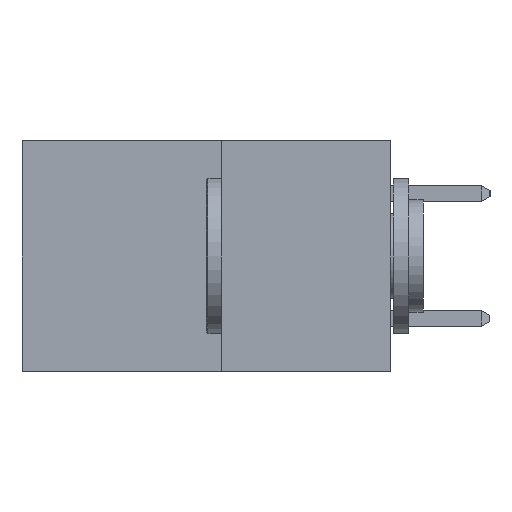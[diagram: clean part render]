
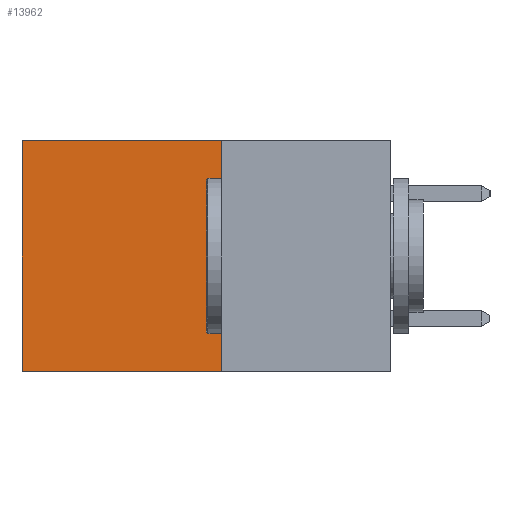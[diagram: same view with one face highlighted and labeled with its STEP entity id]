
A CAD part, left-side view. The second image highlights one B-rep face of the part: STEP entity #13962.
In plain terms, the highlighted planar face has unit normal (-1, 0, 0).
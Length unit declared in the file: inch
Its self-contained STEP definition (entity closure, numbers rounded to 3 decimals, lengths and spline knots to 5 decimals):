
#373 = PLANE ( 'NONE',  #20520 ) ;
#533 = LINE ( 'NONE', #15297, #5423 ) ;
#648 = DIRECTION ( 'NONE',  ( 0., 1., 0. ) ) ;
#1032 = CARTESIAN_POINT ( 'NONE',  ( 0.277, 0.27, -0.37 ) ) ;
#1440 = CARTESIAN_POINT ( 'NONE',  ( 0.277, 0.27, -0.37 ) ) ;
#1794 = ORIENTED_EDGE ( 'NONE', *, *, #9398, .F. ) ;
#2177 = VERTEX_POINT ( 'NONE', #14330 ) ;
#2356 = VECTOR ( 'NONE', #13836, 39.37008 ) ;
#4237 = VERTEX_POINT ( 'NONE', #17198 ) ;
#4848 = ORIENTED_EDGE ( 'NONE', *, *, #15363, .T. ) ;
#5423 = VECTOR ( 'NONE', #17040, 39.37008 ) ;
#5927 = DIRECTION ( 'NONE',  ( 1., 0., 0. ) ) ;
#6181 = EDGE_LOOP ( 'NONE', ( #23161, #22148, #1794, #4848 ) ) ;
#6646 = LINE ( 'NONE', #1032, #2356 ) ;
#6911 = LINE ( 'NONE', #13453, #21367 ) ;
#7151 = LINE ( 'NONE', #15505, #11438 ) ;
#9398 = EDGE_CURVE ( 'NONE', #4237, #13643, #6646, .T. ) ;
#11438 = VECTOR ( 'NONE', #19199, 39.37008 ) ;
#11523 = EDGE_CURVE ( 'NONE', #2177, #14095, #7151, .T. ) ;
#13314 = FACE_OUTER_BOUND ( 'NONE', #6181, .T. ) ;
#13453 = CARTESIAN_POINT ( 'NONE',  ( 0.277, 0.27, 0. ) ) ;
#13643 = VERTEX_POINT ( 'NONE', #1440 ) ;
#13836 = DIRECTION ( 'NONE',  ( 0., 0., -1. ) ) ;
#13962 = ADVANCED_FACE ( 'NONE', ( #13314 ), #373, .F. ) ;
#14095 = VERTEX_POINT ( 'NONE', #18952 ) ;
#14330 = CARTESIAN_POINT ( 'NONE',  ( 0.277, 0.59, 0. ) ) ;
#15297 = CARTESIAN_POINT ( 'NONE',  ( 0.277, 0.27, -0.37 ) ) ;
#15363 = EDGE_CURVE ( 'NONE', #4237, #2177, #6911, .T. ) ;
#15505 = CARTESIAN_POINT ( 'NONE',  ( 0.277, 0.59, -0.37 ) ) ;
#16847 = CARTESIAN_POINT ( 'NONE',  ( 0.277, 0.27, -0.37 ) ) ;
#17040 = DIRECTION ( 'NONE',  ( 0., 1., 0. ) ) ;
#17198 = CARTESIAN_POINT ( 'NONE',  ( 0.277, 0.27, 0. ) ) ;
#17203 = EDGE_CURVE ( 'NONE', #13643, #14095, #533, .T. ) ;
#18659 = DIRECTION ( 'NONE',  ( 0., 0., -1. ) ) ;
#18952 = CARTESIAN_POINT ( 'NONE',  ( 0.277, 0.59, -0.37 ) ) ;
#19199 = DIRECTION ( 'NONE',  ( 0., 0., -1. ) ) ;
#20520 = AXIS2_PLACEMENT_3D ( 'NONE', #16847, #5927, #18659 ) ;
#21367 = VECTOR ( 'NONE', #648, 39.37008 ) ;
#22148 = ORIENTED_EDGE ( 'NONE', *, *, #17203, .F. ) ;
#23161 = ORIENTED_EDGE ( 'NONE', *, *, #11523, .T. ) ;
